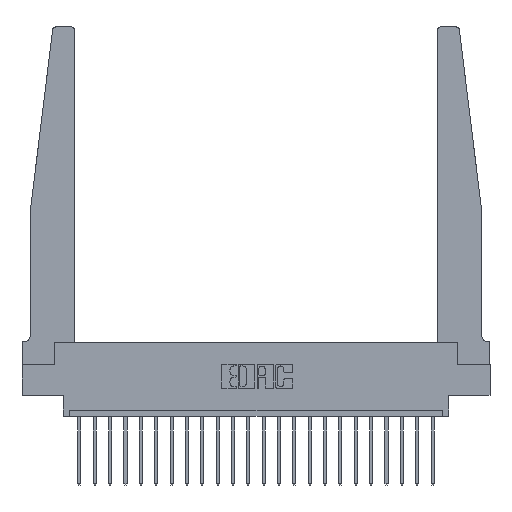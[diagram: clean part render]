
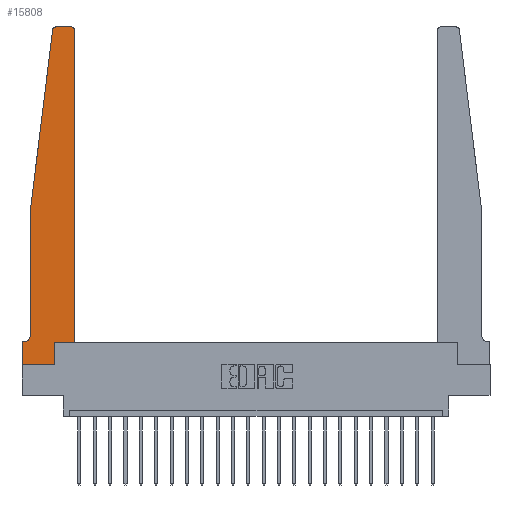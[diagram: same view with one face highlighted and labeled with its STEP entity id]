
A CAD part, top view. The second image highlights one B-rep face of the part: STEP entity #15808.
In plain terms, the highlighted planar face has unit normal (0, 0, 1).
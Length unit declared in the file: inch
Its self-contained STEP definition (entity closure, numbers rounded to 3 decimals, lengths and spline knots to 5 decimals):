
#310 = CIRCLE ( 'NONE', #10162, 0.05 ) ;
#586 = DIRECTION ( 'NONE',  ( 0., -1., 0. ) ) ;
#655 = CARTESIAN_POINT ( 'NONE',  ( 0.425, 0.18, 0.37 ) ) ;
#661 = EDGE_CURVE ( 'NONE', #15271, #3306, #15352, .T. ) ;
#971 = EDGE_LOOP ( 'NONE', ( #3822, #8345, #1836, #1314, #5623, #7718, #1606, #17846, #1602, #12997, #5440, #11216 ) ) ;
#1006 = CARTESIAN_POINT ( 'NONE',  ( 0.065, 1.25, 0.37 ) ) ;
#1314 = ORIENTED_EDGE ( 'NONE', *, *, #5664, .T. ) ;
#1375 = LINE ( 'NONE', #8590, #16826 ) ;
#1602 = ORIENTED_EDGE ( 'NONE', *, *, #3932, .T. ) ;
#1606 = ORIENTED_EDGE ( 'NONE', *, *, #21646, .T. ) ;
#1691 = DIRECTION ( 'NONE',  ( 0., 0., 1. ) ) ;
#1727 = CARTESIAN_POINT ( 'NONE',  ( 0.065, 1.25, 0.37 ) ) ;
#1836 = ORIENTED_EDGE ( 'NONE', *, *, #22223, .T. ) ;
#2174 = LINE ( 'NONE', #21783, #4313 ) ;
#2385 = EDGE_CURVE ( 'NONE', #16338, #4436, #15476, .T. ) ;
#2790 = EDGE_CURVE ( 'NONE', #4960, #19219, #11988, .T. ) ;
#2913 = CARTESIAN_POINT ( 'NONE',  ( 0.065, 0.1875, 0.37 ) ) ;
#3114 = DIRECTION ( 'NONE',  ( 1., 0., 0. ) ) ;
#3306 = VERTEX_POINT ( 'NONE', #21374 ) ;
#3378 = DIRECTION ( 'NONE',  ( -1., 0., 0. ) ) ;
#3593 = CARTESIAN_POINT ( 'NONE',  ( 0.065, 0.2375, 0.37 ) ) ;
#3675 = VECTOR ( 'NONE', #586, 39.37008 ) ;
#3822 = ORIENTED_EDGE ( 'NONE', *, *, #661, .T. ) ;
#3932 = EDGE_CURVE ( 'NONE', #4436, #18009, #2174, .T. ) ;
#4313 = VECTOR ( 'NONE', #14429, 39.37008 ) ;
#4436 = VERTEX_POINT ( 'NONE', #9129 ) ;
#4561 = VECTOR ( 'NONE', #21904, 39.37008 ) ;
#4775 = FACE_OUTER_BOUND ( 'NONE', #971, .T. ) ;
#4938 = VECTOR ( 'NONE', #9769, 39.37008 ) ;
#4960 = VERTEX_POINT ( 'NONE', #22035 ) ;
#4962 = CARTESIAN_POINT ( 'NONE',  ( 0., 0., 0.37 ) ) ;
#5187 = CIRCLE ( 'NONE', #6274, 0.03 ) ;
#5365 = CIRCLE ( 'NONE', #8643, 0.03 ) ;
#5391 = CARTESIAN_POINT ( 'NONE',  ( 0.395, 2.75, 0.37 ) ) ;
#5440 = ORIENTED_EDGE ( 'NONE', *, *, #10974, .T. ) ;
#5523 = VERTEX_POINT ( 'NONE', #14802 ) ;
#5580 = CARTESIAN_POINT ( 'NONE',  ( 0., 0.1875, 0.37 ) ) ;
#5623 = ORIENTED_EDGE ( 'NONE', *, *, #17794, .T. ) ;
#5664 = EDGE_CURVE ( 'NONE', #6294, #10912, #8955, .T. ) ;
#5924 = EDGE_CURVE ( 'NONE', #18009, #10514, #1375, .T. ) ;
#6250 = VECTOR ( 'NONE', #12504, 39.37008 ) ;
#6274 = AXIS2_PLACEMENT_3D ( 'NONE', #18483, #9760, #3114 ) ;
#6294 = VERTEX_POINT ( 'NONE', #1006 ) ;
#6486 = CARTESIAN_POINT ( 'NONE',  ( 0.015, 0.2375, 0.37 ) ) ;
#6708 = VECTOR ( 'NONE', #10914, 39.37008 ) ;
#7119 = LINE ( 'NONE', #1727, #6250 ) ;
#7160 = LINE ( 'NONE', #21161, #6708 ) ;
#7467 = CARTESIAN_POINT ( 'NONE',  ( 0.065, 1.25, 0.37 ) ) ;
#7718 = ORIENTED_EDGE ( 'NONE', *, *, #2790, .T. ) ;
#8136 = CARTESIAN_POINT ( 'NONE',  ( 0., 0., 0.37 ) ) ;
#8345 = ORIENTED_EDGE ( 'NONE', *, *, #21641, .T. ) ;
#8590 = CARTESIAN_POINT ( 'NONE',  ( 0.425, 0.18, 0.37 ) ) ;
#8639 = DIRECTION ( 'NONE',  ( 0., 0., 1. ) ) ;
#8643 = AXIS2_PLACEMENT_3D ( 'NONE', #15521, #8639, #22193 ) ;
#8955 = LINE ( 'NONE', #7467, #3675 ) ;
#9129 = CARTESIAN_POINT ( 'NONE',  ( 0.2605, 0., 0.37 ) ) ;
#9760 = DIRECTION ( 'NONE',  ( 0., 0., 1. ) ) ;
#9769 = DIRECTION ( 'NONE',  ( -1., 0., 0. ) ) ;
#9910 = DIRECTION ( 'NONE',  ( -1., 0., 0. ) ) ;
#10071 = DIRECTION ( 'NONE',  ( 1., 0., 0. ) ) ;
#10132 = DIRECTION ( 'NONE',  ( 0., 0., -1. ) ) ;
#10162 = AXIS2_PLACEMENT_3D ( 'NONE', #6486, #10132, #9910 ) ;
#10385 = CARTESIAN_POINT ( 'NONE',  ( 0., 0.1875, 0.37 ) ) ;
#10454 = DIRECTION ( 'NONE',  ( 0., -1., 0. ) ) ;
#10514 = VERTEX_POINT ( 'NONE', #655 ) ;
#10912 = VERTEX_POINT ( 'NONE', #3593 ) ;
#10914 = DIRECTION ( 'NONE',  ( 0., 1., 0. ) ) ;
#10974 = EDGE_CURVE ( 'NONE', #10514, #5523, #7160, .T. ) ;
#11216 = ORIENTED_EDGE ( 'NONE', *, *, #16129, .T. ) ;
#11848 = LINE ( 'NONE', #4962, #22023 ) ;
#11988 = LINE ( 'NONE', #2913, #18664 ) ;
#12248 = DIRECTION ( 'NONE',  ( 1., 0., 0. ) ) ;
#12305 = AXIS2_PLACEMENT_3D ( 'NONE', #10385, #1691, #12248 ) ;
#12504 = DIRECTION ( 'NONE',  ( -0.122, -0.992, 0. ) ) ;
#12997 = ORIENTED_EDGE ( 'NONE', *, *, #5924, .T. ) ;
#13230 = VERTEX_POINT ( 'NONE', #15511 ) ;
#14249 = CARTESIAN_POINT ( 'NONE',  ( 0., 0., 0.37 ) ) ;
#14429 = DIRECTION ( 'NONE',  ( 0., 1., 0. ) ) ;
#14802 = CARTESIAN_POINT ( 'NONE',  ( 0.425, 2.72, 0.37 ) ) ;
#15271 = VERTEX_POINT ( 'NONE', #5391 ) ;
#15352 = LINE ( 'NONE', #21837, #4938 ) ;
#15476 = LINE ( 'NONE', #8136, #4561 ) ;
#15511 = CARTESIAN_POINT ( 'NONE',  ( 0.24675, 2.72367, 0.37 ) ) ;
#15521 = CARTESIAN_POINT ( 'NONE',  ( 0.395, 2.72, 0.37 ) ) ;
#15808 = ADVANCED_FACE ( 'NONE', ( #4775 ), #17499, .T. ) ;
#15880 = CARTESIAN_POINT ( 'NONE',  ( 0.2605, 0.18, 0.37 ) ) ;
#16129 = EDGE_CURVE ( 'NONE', #5523, #15271, #5365, .T. ) ;
#16338 = VERTEX_POINT ( 'NONE', #14249 ) ;
#16826 = VECTOR ( 'NONE', #10071, 39.37008 ) ;
#17499 = PLANE ( 'NONE',  #12305 ) ;
#17794 = EDGE_CURVE ( 'NONE', #10912, #4960, #310, .T. ) ;
#17846 = ORIENTED_EDGE ( 'NONE', *, *, #2385, .T. ) ;
#18009 = VERTEX_POINT ( 'NONE', #15880 ) ;
#18483 = CARTESIAN_POINT ( 'NONE',  ( 0.27653, 2.72, 0.37 ) ) ;
#18664 = VECTOR ( 'NONE', #3378, 39.37008 ) ;
#19219 = VERTEX_POINT ( 'NONE', #5580 ) ;
#21161 = CARTESIAN_POINT ( 'NONE',  ( 0.425, 0.18, 0.37 ) ) ;
#21374 = CARTESIAN_POINT ( 'NONE',  ( 0.27653, 2.75, 0.37 ) ) ;
#21641 = EDGE_CURVE ( 'NONE', #3306, #13230, #5187, .T. ) ;
#21646 = EDGE_CURVE ( 'NONE', #19219, #16338, #11848, .T. ) ;
#21783 = CARTESIAN_POINT ( 'NONE',  ( 0.2605, 0.18, 0.37 ) ) ;
#21837 = CARTESIAN_POINT ( 'NONE',  ( 0.25, 2.75, 0.37 ) ) ;
#21904 = DIRECTION ( 'NONE',  ( 1., 0., 0. ) ) ;
#22023 = VECTOR ( 'NONE', #10454, 39.37008 ) ;
#22035 = CARTESIAN_POINT ( 'NONE',  ( 0.015, 0.1875, 0.37 ) ) ;
#22193 = DIRECTION ( 'NONE',  ( 1., 0., 0. ) ) ;
#22223 = EDGE_CURVE ( 'NONE', #13230, #6294, #7119, .T. ) ;
